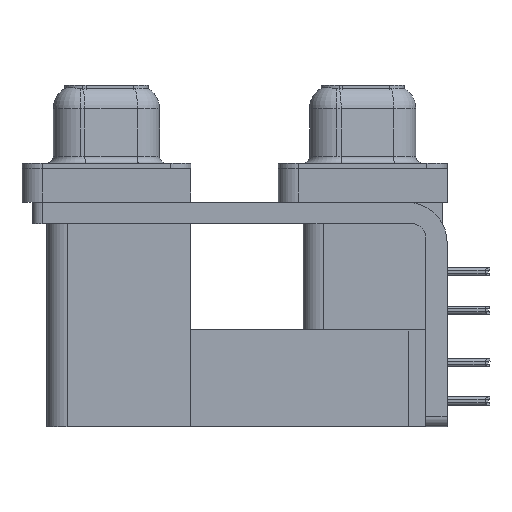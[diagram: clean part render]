
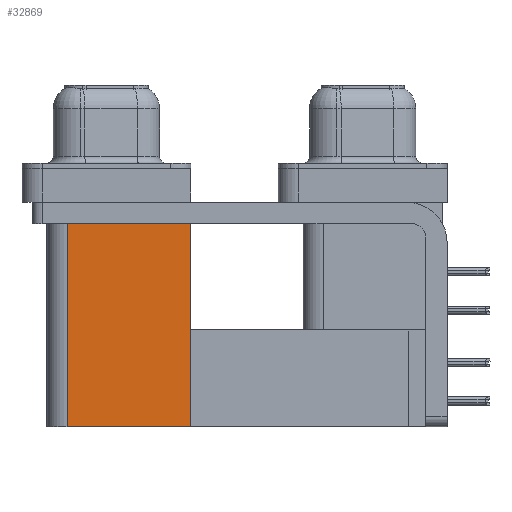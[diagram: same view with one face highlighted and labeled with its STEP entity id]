
A CAD part, left-side view. The second image highlights one B-rep face of the part: STEP entity #32869.
In plain terms, the highlighted planar face has unit normal (-1, 0, 0).
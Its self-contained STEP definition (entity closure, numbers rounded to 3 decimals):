
#920 = VERTEX_POINT ( 'NONE', #25600 ) ;
#1867 = PLANE ( 'NONE',  #18849 ) ;
#1925 = VERTEX_POINT ( 'NONE', #22695 ) ;
#2466 = EDGE_CURVE ( 'NONE', #25770, #22991, #39630, .T. ) ;
#4454 = DIRECTION ( 'NONE',  ( 0., 1., 0. ) ) ;
#4948 = DIRECTION ( 'NONE',  ( 1., 0., 0. ) ) ;
#6716 = EDGE_CURVE ( 'NONE', #1925, #25770, #12200, .T. ) ;
#7736 = CARTESIAN_POINT ( 'NONE',  ( 3.765, 21.975, -2.5 ) ) ;
#9412 = FACE_OUTER_BOUND ( 'NONE', #18501, .T. ) ;
#9582 = EDGE_CURVE ( 'NONE', #920, #22991, #21053, .T. ) ;
#12200 = LINE ( 'NONE', #40774, #36539 ) ;
#16239 = CARTESIAN_POINT ( 'NONE',  ( 3.765, 21.975, -19.2 ) ) ;
#18501 = EDGE_LOOP ( 'NONE', ( #22541, #45863, #44865, #21626 ) ) ;
#18593 = LINE ( 'NONE', #39210, #20734 ) ;
#18849 = AXIS2_PLACEMENT_3D ( 'NONE', #30979, #4948, #23482 ) ;
#19477 = VECTOR ( 'NONE', #4454, 1000. ) ;
#20734 = VECTOR ( 'NONE', #32171, 1000. ) ;
#21053 = LINE ( 'NONE', #16239, #22483 ) ;
#21626 = ORIENTED_EDGE ( 'NONE', *, *, #6716, .T. ) ;
#22483 = VECTOR ( 'NONE', #27010, 1000. ) ;
#22541 = ORIENTED_EDGE ( 'NONE', *, *, #2466, .T. ) ;
#22695 = CARTESIAN_POINT ( 'NONE',  ( 3.765, 12.775, -19.2 ) ) ;
#22991 = VERTEX_POINT ( 'NONE', #7736 ) ;
#23482 = DIRECTION ( 'NONE',  ( 0., 0., -1. ) ) ;
#25600 = CARTESIAN_POINT ( 'NONE',  ( 3.765, 21.975, -19.2 ) ) ;
#25770 = VERTEX_POINT ( 'NONE', #27589 ) ;
#26471 = DIRECTION ( 'NONE',  ( 0., 0., 1. ) ) ;
#27010 = DIRECTION ( 'NONE',  ( 0., 0., 1. ) ) ;
#27589 = CARTESIAN_POINT ( 'NONE',  ( 3.765, 12.775, -2.5 ) ) ;
#30034 = CARTESIAN_POINT ( 'NONE',  ( 3.765, 12.775, -2.5 ) ) ;
#30979 = CARTESIAN_POINT ( 'NONE',  ( 3.765, 12.775, -19.2 ) ) ;
#32171 = DIRECTION ( 'NONE',  ( 0., 1., 0. ) ) ;
#32869 = ADVANCED_FACE ( 'NONE', ( #9412 ), #1867, .F. ) ;
#36539 = VECTOR ( 'NONE', #26471, 1000. ) ;
#39210 = CARTESIAN_POINT ( 'NONE',  ( 3.765, 12.775, -19.2 ) ) ;
#39630 = LINE ( 'NONE', #30034, #19477 ) ;
#40774 = CARTESIAN_POINT ( 'NONE',  ( 3.765, 12.775, -19.2 ) ) ;
#44544 = EDGE_CURVE ( 'NONE', #1925, #920, #18593, .T. ) ;
#44865 = ORIENTED_EDGE ( 'NONE', *, *, #44544, .F. ) ;
#45863 = ORIENTED_EDGE ( 'NONE', *, *, #9582, .F. ) ;
